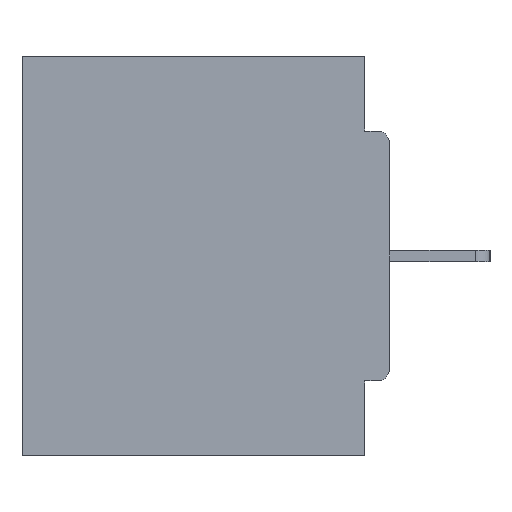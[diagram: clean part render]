
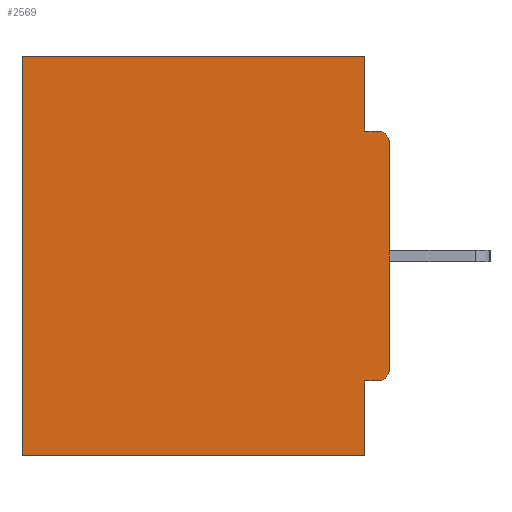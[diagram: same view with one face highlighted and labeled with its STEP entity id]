
A CAD part, left-side view. The second image highlights one B-rep face of the part: STEP entity #2569.
In plain terms, the highlighted planar face has unit normal (-1, 0, 0).
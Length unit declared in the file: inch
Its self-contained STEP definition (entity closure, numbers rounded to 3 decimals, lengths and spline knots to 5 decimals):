
#33 = CARTESIAN_POINT ( 'NONE',  ( 0.298, 0.015, -0.3915 ) ) ;
#588 = CARTESIAN_POINT ( 'NONE',  ( 0.298, 0.015, -0.1085 ) ) ;
#1279 = CARTESIAN_POINT ( 'NONE',  ( 0.298, 0.031, -0.5 ) ) ;
#1322 = ORIENTED_EDGE ( 'NONE', *, *, #18086, .T. ) ;
#1405 = CARTESIAN_POINT ( 'NONE',  ( 0.298, 0.031, 0. ) ) ;
#1565 = CARTESIAN_POINT ( 'NONE',  ( 0.298, 0.46, 0. ) ) ;
#1581 = DIRECTION ( 'NONE',  ( 1., 0., 0. ) ) ;
#2379 = DIRECTION ( 'NONE',  ( -1., 0., 0. ) ) ;
#2569 = ADVANCED_FACE ( 'NONE', ( #27620 ), #17815, .F. ) ;
#3285 = DIRECTION ( 'NONE',  ( 0., 0., -1. ) ) ;
#4203 = LINE ( 'NONE', #13415, #23132 ) ;
#4273 = LINE ( 'NONE', #25926, #15103 ) ;
#4345 = EDGE_CURVE ( 'NONE', #27243, #6720, #29249, .T. ) ;
#5151 = EDGE_CURVE ( 'NONE', #27243, #21979, #19656, .T. ) ;
#5216 = EDGE_CURVE ( 'NONE', #23122, #18307, #4203, .T. ) ;
#6608 = EDGE_CURVE ( 'NONE', #13783, #23122, #25712, .T. ) ;
#6629 = ORIENTED_EDGE ( 'NONE', *, *, #23582, .F. ) ;
#6720 = VERTEX_POINT ( 'NONE', #21042 ) ;
#6812 = CARTESIAN_POINT ( 'NONE',  ( 0.298, 0.46, 0. ) ) ;
#7121 = VECTOR ( 'NONE', #7426, 39.37008 ) ;
#7179 = ORIENTED_EDGE ( 'NONE', *, *, #5151, .F. ) ;
#7357 = CARTESIAN_POINT ( 'NONE',  ( 0.298, 0.031, -0.0935 ) ) ;
#7426 = DIRECTION ( 'NONE',  ( 0., 0., -1. ) ) ;
#7787 = LINE ( 'NONE', #26488, #17044 ) ;
#8380 = DIRECTION ( 'NONE',  ( 0., 0., -1. ) ) ;
#8785 = CARTESIAN_POINT ( 'NONE',  ( 0.298, 0., -0.5 ) ) ;
#9012 = LINE ( 'NONE', #25684, #11745 ) ;
#9062 = VECTOR ( 'NONE', #23978, 39.37008 ) ;
#9101 = DIRECTION ( 'NONE',  ( 0., 1., 0. ) ) ;
#9831 = EDGE_CURVE ( 'NONE', #28430, #6720, #9012, .T. ) ;
#10586 = CARTESIAN_POINT ( 'NONE',  ( 0.298, 0., 0. ) ) ;
#11042 = ORIENTED_EDGE ( 'NONE', *, *, #5216, .F. ) ;
#11745 = VECTOR ( 'NONE', #18681, 39.37008 ) ;
#11875 = DIRECTION ( 'NONE',  ( 0., 0., -1. ) ) ;
#13252 = ORIENTED_EDGE ( 'NONE', *, *, #25620, .T. ) ;
#13320 = VECTOR ( 'NONE', #3285, 39.37008 ) ;
#13415 = CARTESIAN_POINT ( 'NONE',  ( 0.298, 0.031, -0.5 ) ) ;
#13783 = VERTEX_POINT ( 'NONE', #18329 ) ;
#15103 = VECTOR ( 'NONE', #9101, 39.37008 ) ;
#15477 = EDGE_CURVE ( 'NONE', #18307, #22173, #29830, .T. ) ;
#15561 = CIRCLE ( 'NONE', #22030, 0.015 ) ;
#15940 = CARTESIAN_POINT ( 'NONE',  ( 0.298, 0., 0. ) ) ;
#17044 = VECTOR ( 'NONE', #28985, 39.37008 ) ;
#17283 = DIRECTION ( 'NONE',  ( -1., 0., 0. ) ) ;
#17815 = PLANE ( 'NONE',  #25676 ) ;
#18086 = EDGE_CURVE ( 'NONE', #20082, #23291, #4273, .T. ) ;
#18307 = VERTEX_POINT ( 'NONE', #1279 ) ;
#18329 = CARTESIAN_POINT ( 'NONE',  ( 0.298, 0.015, -0.4065 ) ) ;
#18400 = DIRECTION ( 'NONE',  ( 0., 0., -1. ) ) ;
#18681 = DIRECTION ( 'NONE',  ( 0., -1., 0. ) ) ;
#19656 = LINE ( 'NONE', #10586, #13320 ) ;
#20012 = ORIENTED_EDGE ( 'NONE', *, *, #4345, .T. ) ;
#20082 = VERTEX_POINT ( 'NONE', #1405 ) ;
#20599 = DIRECTION ( 'NONE',  ( 0., 0., -1. ) ) ;
#20675 = EDGE_CURVE ( 'NONE', #13783, #21979, #15561, .T. ) ;
#20942 = ORIENTED_EDGE ( 'NONE', *, *, #9831, .F. ) ;
#21042 = CARTESIAN_POINT ( 'NONE',  ( 0.298, 0.015, -0.0935 ) ) ;
#21859 = CARTESIAN_POINT ( 'NONE',  ( 0.298, 0.031, -0.4065 ) ) ;
#21979 = VERTEX_POINT ( 'NONE', #26517 ) ;
#22030 = AXIS2_PLACEMENT_3D ( 'NONE', #33, #2379, #11875 ) ;
#22173 = VERTEX_POINT ( 'NONE', #25556 ) ;
#22507 = DIRECTION ( 'NONE',  ( 0., 1., 0. ) ) ;
#22845 = CARTESIAN_POINT ( 'NONE',  ( 0.298, 0., -0.1085 ) ) ;
#23122 = VERTEX_POINT ( 'NONE', #21859 ) ;
#23132 = VECTOR ( 'NONE', #18400, 39.37008 ) ;
#23291 = VERTEX_POINT ( 'NONE', #1565 ) ;
#23528 = CARTESIAN_POINT ( 'NONE',  ( 0.298, 0., -0.4065 ) ) ;
#23582 = EDGE_CURVE ( 'NONE', #20082, #28430, #7787, .T. ) ;
#23978 = DIRECTION ( 'NONE',  ( 0., 1., 0. ) ) ;
#25556 = CARTESIAN_POINT ( 'NONE',  ( 0.298, 0.46, -0.5 ) ) ;
#25620 = EDGE_CURVE ( 'NONE', #23291, #22173, #28170, .T. ) ;
#25676 = AXIS2_PLACEMENT_3D ( 'NONE', #15940, #1581, #20599 ) ;
#25684 = CARTESIAN_POINT ( 'NONE',  ( 0.298, 0., -0.0935 ) ) ;
#25712 = LINE ( 'NONE', #23528, #9062 ) ;
#25732 = EDGE_LOOP ( 'NONE', ( #20012, #20942, #6629, #1322, #13252, #29400, #11042, #30144, #28541, #7179 ) ) ;
#25926 = CARTESIAN_POINT ( 'NONE',  ( 0.298, 0., 0. ) ) ;
#26488 = CARTESIAN_POINT ( 'NONE',  ( 0.298, 0.031, -0.5 ) ) ;
#26517 = CARTESIAN_POINT ( 'NONE',  ( 0.298, 0., -0.3915 ) ) ;
#27243 = VERTEX_POINT ( 'NONE', #22845 ) ;
#27620 = FACE_OUTER_BOUND ( 'NONE', #25732, .T. ) ;
#27760 = AXIS2_PLACEMENT_3D ( 'NONE', #588, #17283, #8380 ) ;
#28170 = LINE ( 'NONE', #6812, #7121 ) ;
#28430 = VERTEX_POINT ( 'NONE', #7357 ) ;
#28541 = ORIENTED_EDGE ( 'NONE', *, *, #20675, .T. ) ;
#28985 = DIRECTION ( 'NONE',  ( 0., 0., -1. ) ) ;
#29249 = CIRCLE ( 'NONE', #27760, 0.015 ) ;
#29400 = ORIENTED_EDGE ( 'NONE', *, *, #15477, .F. ) ;
#29830 = LINE ( 'NONE', #8785, #30331 ) ;
#30144 = ORIENTED_EDGE ( 'NONE', *, *, #6608, .F. ) ;
#30331 = VECTOR ( 'NONE', #22507, 39.37008 ) ;
